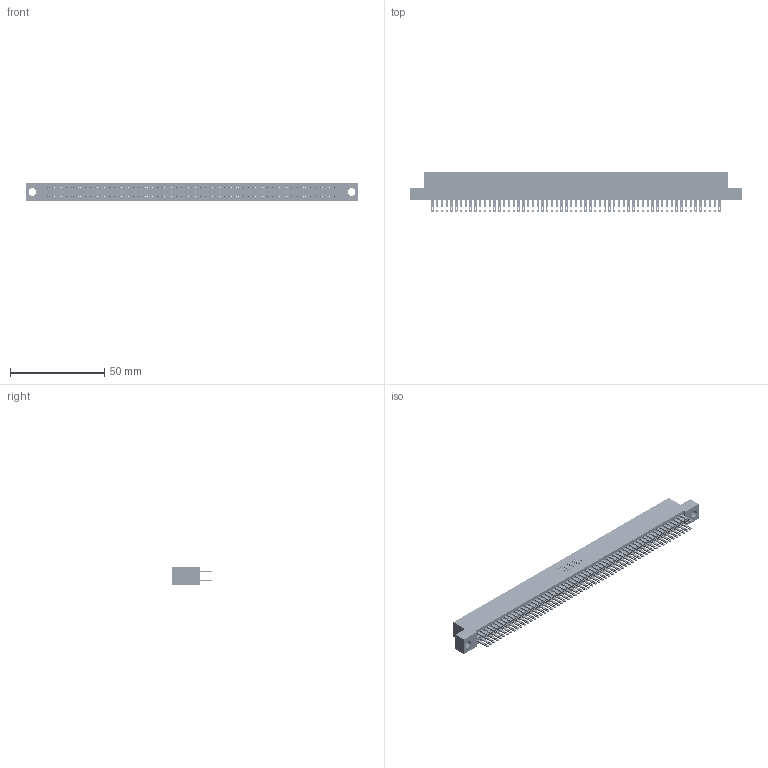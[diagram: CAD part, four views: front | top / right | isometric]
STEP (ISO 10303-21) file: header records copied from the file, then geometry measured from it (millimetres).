
FILE_DESCRIPTION (( 'STEP AP203' ), '1' );
FILE_NAME ('345-122-500-204.STEP', '2021-05-25T17:20:26', ( '' ), ( '' ), 'SwSTEP 2.0', 'SolidWorks 2020', '' );
FILE_SCHEMA (( 'CONFIG_CONTROL_DESIGN' ));
Length unit declared in the file: inch
Products named in the file (3): 345-292-001_345-293-100; 345 Part_Flush Mounting Lugs - 0.156 Dia-TI; 345-122-500-204
Assembly tree (123 placements, depth 2):
  345-122-500-204
    345 Part_Flush Mounting Lugs - 0.156 Dia-TI
    345-292-001_345-293-100  x122
Bounding box: 176.15 x 21.51 x 9.4 mm (x, y, z)
Volume: 17554.5 mm3; surface area: 27412.4 mm2
Topology: 123 solids, 123 shells, 5752 faces, 17579 edges, 11718 vertices
Faces by surface type: plane 3388, cylinder 2364
Entity records: 45653 total; most frequent: CARTESIAN_POINT 7638, ORIENTED_EDGE 7570, DIRECTION 6713, EDGE_CURVE 3785, VECTOR 3405, LINE 3405, VERTEX_POINT 2522, AXIS2_PLACEMENT_3D 1654
